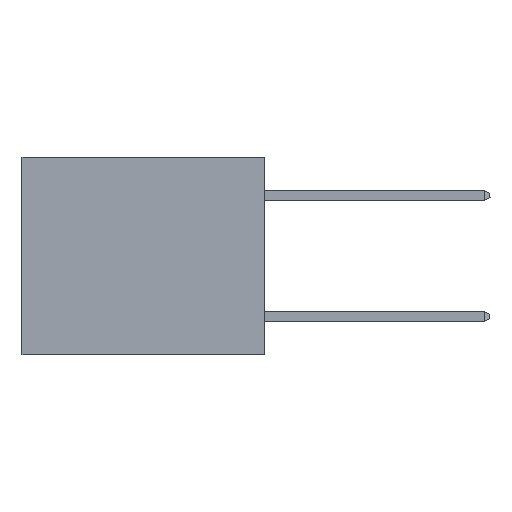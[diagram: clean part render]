
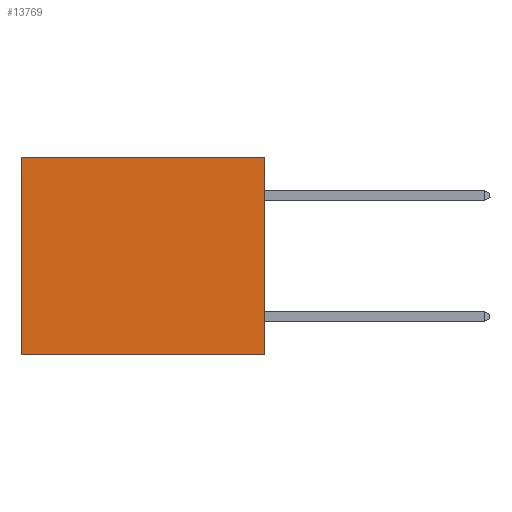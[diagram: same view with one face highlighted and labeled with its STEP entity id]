
A CAD part, left-side view. The second image highlights one B-rep face of the part: STEP entity #13769.
In plain terms, the highlighted planar face has unit normal (-1, 0, 0).
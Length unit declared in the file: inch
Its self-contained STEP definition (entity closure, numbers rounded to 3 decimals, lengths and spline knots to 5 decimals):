
#215 = CARTESIAN_POINT ( 'NONE',  ( 0.3165, 0., -0.49 ) ) ;
#969 = LINE ( 'NONE', #30088, #2970 ) ;
#1217 = FACE_OUTER_BOUND ( 'NONE', #12489, .T. ) ;
#2453 = ORIENTED_EDGE ( 'NONE', *, *, #33454, .T. ) ;
#2827 = ORIENTED_EDGE ( 'NONE', *, *, #29395, .F. ) ;
#2970 = VECTOR ( 'NONE', #32713, 39.37008 ) ;
#4152 = PLANE ( 'NONE',  #26735 ) ;
#4532 = CARTESIAN_POINT ( 'NONE',  ( 0.3165, 0.6, -0.49 ) ) ;
#6466 = VERTEX_POINT ( 'NONE', #17733 ) ;
#6817 = LINE ( 'NONE', #27147, #17666 ) ;
#7517 = EDGE_CURVE ( 'NONE', #6466, #23361, #18751, .T. ) ;
#10084 = CARTESIAN_POINT ( 'NONE',  ( 0.3165, 0., -0.49 ) ) ;
#12489 = EDGE_LOOP ( 'NONE', ( #2453, #2827, #26773, #26859 ) ) ;
#13456 = VECTOR ( 'NONE', #33198, 39.37008 ) ;
#13769 = ADVANCED_FACE ( 'NONE', ( #1217 ), #4152, .F. ) ;
#15124 = CARTESIAN_POINT ( 'NONE',  ( 0.3165, 0.6, 0. ) ) ;
#16849 = DIRECTION ( 'NONE',  ( 0., 1., 0. ) ) ;
#17666 = VECTOR ( 'NONE', #16849, 39.37008 ) ;
#17733 = CARTESIAN_POINT ( 'NONE',  ( 0.3165, 0., 0. ) ) ;
#18751 = LINE ( 'NONE', #10084, #19966 ) ;
#19966 = VECTOR ( 'NONE', #28127, 39.37008 ) ;
#20294 = LINE ( 'NONE', #25364, #13456 ) ;
#22100 = DIRECTION ( 'NONE',  ( 0., 0., -1. ) ) ;
#22552 = DIRECTION ( 'NONE',  ( 1., 0., 0. ) ) ;
#23361 = VERTEX_POINT ( 'NONE', #215 ) ;
#24016 = VERTEX_POINT ( 'NONE', #15124 ) ;
#24925 = CARTESIAN_POINT ( 'NONE',  ( 0.3165, 0., -0.49 ) ) ;
#25364 = CARTESIAN_POINT ( 'NONE',  ( 0.3165, 0., -0.49 ) ) ;
#26735 = AXIS2_PLACEMENT_3D ( 'NONE', #24925, #22552, #22100 ) ;
#26773 = ORIENTED_EDGE ( 'NONE', *, *, #7517, .F. ) ;
#26859 = ORIENTED_EDGE ( 'NONE', *, *, #30096, .T. ) ;
#27147 = CARTESIAN_POINT ( 'NONE',  ( 0.3165, 0., 0. ) ) ;
#28127 = DIRECTION ( 'NONE',  ( 0., 0., -1. ) ) ;
#29395 = EDGE_CURVE ( 'NONE', #23361, #33369, #20294, .T. ) ;
#30088 = CARTESIAN_POINT ( 'NONE',  ( 0.3165, 0.6, -0.49 ) ) ;
#30096 = EDGE_CURVE ( 'NONE', #6466, #24016, #6817, .T. ) ;
#32713 = DIRECTION ( 'NONE',  ( 0., 0., -1. ) ) ;
#33198 = DIRECTION ( 'NONE',  ( 0., 1., 0. ) ) ;
#33369 = VERTEX_POINT ( 'NONE', #4532 ) ;
#33454 = EDGE_CURVE ( 'NONE', #24016, #33369, #969, .T. ) ;
